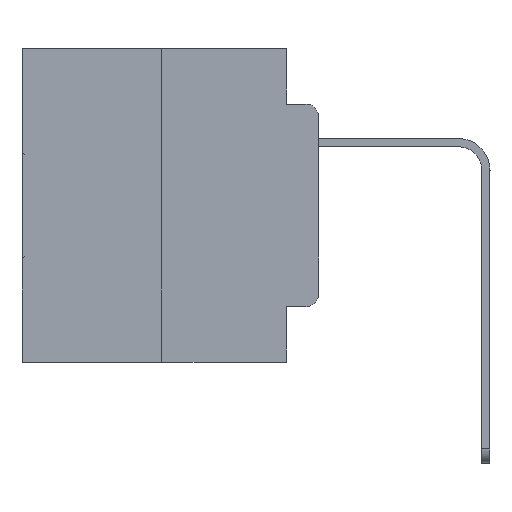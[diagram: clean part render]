
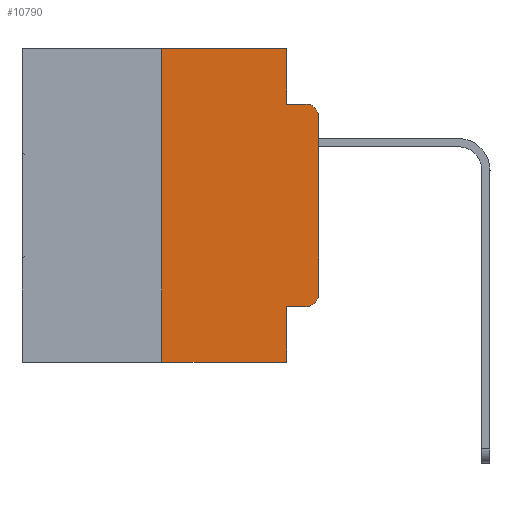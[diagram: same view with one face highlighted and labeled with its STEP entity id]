
A CAD part, left-side view. The second image highlights one B-rep face of the part: STEP entity #10790.
In plain terms, the highlighted planar face has unit normal (-1, 0, 0).
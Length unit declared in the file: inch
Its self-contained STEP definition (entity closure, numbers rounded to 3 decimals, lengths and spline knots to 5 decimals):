
#261 = EDGE_CURVE ( 'NONE', #13056, #20516, #25706, .T. ) ;
#331 = DIRECTION ( 'NONE',  ( 0., -1., 0. ) ) ;
#450 = LINE ( 'NONE', #11831, #4779 ) ;
#1232 = ORIENTED_EDGE ( 'NONE', *, *, #9289, .T. ) ;
#1322 = CARTESIAN_POINT ( 'NONE',  ( 0., 0.051, -0.0885 ) ) ;
#1327 = DIRECTION ( 'NONE',  ( 0., 0., 1. ) ) ;
#1960 = CARTESIAN_POINT ( 'NONE',  ( 0., 0.473, 0. ) ) ;
#2328 = CARTESIAN_POINT ( 'NONE',  ( 0., 0.473, 0. ) ) ;
#2825 = DIRECTION ( 'NONE',  ( 0., 0., 1. ) ) ;
#2968 = CIRCLE ( 'NONE', #25870, 0.02 ) ;
#3244 = DIRECTION ( 'NONE',  ( 0., -1., 0. ) ) ;
#3782 = ORIENTED_EDGE ( 'NONE', *, *, #261, .T. ) ;
#4067 = AXIS2_PLACEMENT_3D ( 'NONE', #21794, #7957, #21689 ) ;
#4076 = DIRECTION ( 'NONE',  ( 0., 0., -1. ) ) ;
#4779 = VECTOR ( 'NONE', #25373, 39.37008 ) ;
#4971 = CIRCLE ( 'NONE', #4067, 0.02 ) ;
#5511 = VERTEX_POINT ( 'NONE', #26132 ) ;
#5815 = AXIS2_PLACEMENT_3D ( 'NONE', #1960, #29541, #8828 ) ;
#6284 = VERTEX_POINT ( 'NONE', #7393 ) ;
#6319 = LINE ( 'NONE', #12357, #19334 ) ;
#7393 = CARTESIAN_POINT ( 'NONE',  ( 0., 0., -0.3915 ) ) ;
#7795 = LINE ( 'NONE', #10802, #28072 ) ;
#7957 = DIRECTION ( 'NONE',  ( -1., 0., 0. ) ) ;
#8068 = CARTESIAN_POINT ( 'NONE',  ( 0., 0.051, -0.5 ) ) ;
#8568 = CARTESIAN_POINT ( 'NONE',  ( 0., 0., -0.1085 ) ) ;
#8631 = CARTESIAN_POINT ( 'NONE',  ( 0., 0.02, -0.1085 ) ) ;
#8828 = DIRECTION ( 'NONE',  ( 0., 0., -1. ) ) ;
#9289 = EDGE_CURVE ( 'NONE', #18850, #25964, #2968, .T. ) ;
#9648 = ORIENTED_EDGE ( 'NONE', *, *, #10209, .T. ) ;
#9759 = ORIENTED_EDGE ( 'NONE', *, *, #24060, .F. ) ;
#10209 = EDGE_CURVE ( 'NONE', #6284, #18850, #12291, .T. ) ;
#10250 = CARTESIAN_POINT ( 'NONE',  ( 0., 0.02, -0.0885 ) ) ;
#10572 = VERTEX_POINT ( 'NONE', #28753 ) ;
#10612 = CARTESIAN_POINT ( 'NONE',  ( 0., 0.051, -0.4115 ) ) ;
#10790 = ADVANCED_FACE ( 'NONE', ( #12600 ), #29660, .F. ) ;
#10802 = CARTESIAN_POINT ( 'NONE',  ( 0., 0.25, 0. ) ) ;
#11635 = LINE ( 'NONE', #2328, #15584 ) ;
#11815 = EDGE_CURVE ( 'NONE', #20516, #6284, #4971, .T. ) ;
#11831 = CARTESIAN_POINT ( 'NONE',  ( 0., 0.051, 0. ) ) ;
#12291 = LINE ( 'NONE', #28083, #13750 ) ;
#12319 = VERTEX_POINT ( 'NONE', #19251 ) ;
#12357 = CARTESIAN_POINT ( 'NONE',  ( 0., 0.051, 0. ) ) ;
#12488 = ORIENTED_EDGE ( 'NONE', *, *, #26448, .F. ) ;
#12600 = FACE_OUTER_BOUND ( 'NONE', #18421, .T. ) ;
#13056 = VERTEX_POINT ( 'NONE', #10612 ) ;
#13747 = ORIENTED_EDGE ( 'NONE', *, *, #19935, .T. ) ;
#13750 = VECTOR ( 'NONE', #2825, 39.37008 ) ;
#14629 = CARTESIAN_POINT ( 'NONE',  ( 0., 0.473, -0.5 ) ) ;
#15311 = ORIENTED_EDGE ( 'NONE', *, *, #15636, .F. ) ;
#15584 = VECTOR ( 'NONE', #331, 39.37008 ) ;
#15636 = EDGE_CURVE ( 'NONE', #10572, #5511, #7795, .T. ) ;
#15738 = ORIENTED_EDGE ( 'NONE', *, *, #23902, .F. ) ;
#16781 = CARTESIAN_POINT ( 'NONE',  ( 0., 0.051, -0.4115 ) ) ;
#16841 = DIRECTION ( 'NONE',  ( 0., -1., 0. ) ) ;
#18421 = EDGE_LOOP ( 'NONE', ( #9648, #1232, #9759, #20560, #15738, #15311, #13747, #12488, #3782, #26384 ) ) ;
#18489 = EDGE_CURVE ( 'NONE', #24319, #12319, #450, .T. ) ;
#18517 = DIRECTION ( 'NONE',  ( 0., 0., -1. ) ) ;
#18850 = VERTEX_POINT ( 'NONE', #8568 ) ;
#19240 = CARTESIAN_POINT ( 'NONE',  ( 0., 0.02, -0.4115 ) ) ;
#19251 = CARTESIAN_POINT ( 'NONE',  ( 0., 0.051, -0.0885 ) ) ;
#19334 = VECTOR ( 'NONE', #18517, 39.37008 ) ;
#19561 = VECTOR ( 'NONE', #23874, 39.37008 ) ;
#19935 = EDGE_CURVE ( 'NONE', #10572, #28666, #22360, .T. ) ;
#20392 = CARTESIAN_POINT ( 'NONE',  ( 0., 0.051, 0. ) ) ;
#20516 = VERTEX_POINT ( 'NONE', #19240 ) ;
#20560 = ORIENTED_EDGE ( 'NONE', *, *, #18489, .F. ) ;
#21689 = DIRECTION ( 'NONE',  ( 0., 0., -1. ) ) ;
#21794 = CARTESIAN_POINT ( 'NONE',  ( 0., 0.02, -0.3915 ) ) ;
#22252 = DIRECTION ( 'NONE',  ( -1., 0., 0. ) ) ;
#22360 = LINE ( 'NONE', #14629, #28887 ) ;
#23874 = DIRECTION ( 'NONE',  ( 0., -1., 0. ) ) ;
#23902 = EDGE_CURVE ( 'NONE', #5511, #24319, #11635, .T. ) ;
#24060 = EDGE_CURVE ( 'NONE', #12319, #25964, #29355, .T. ) ;
#24319 = VERTEX_POINT ( 'NONE', #20392 ) ;
#25373 = DIRECTION ( 'NONE',  ( 0., 0., -1. ) ) ;
#25706 = LINE ( 'NONE', #16781, #19561 ) ;
#25870 = AXIS2_PLACEMENT_3D ( 'NONE', #8631, #22252, #4076 ) ;
#25964 = VERTEX_POINT ( 'NONE', #10250 ) ;
#26132 = CARTESIAN_POINT ( 'NONE',  ( 0., 0.25, 0. ) ) ;
#26384 = ORIENTED_EDGE ( 'NONE', *, *, #11815, .T. ) ;
#26448 = EDGE_CURVE ( 'NONE', #13056, #28666, #6319, .T. ) ;
#27163 = VECTOR ( 'NONE', #3244, 39.37008 ) ;
#28072 = VECTOR ( 'NONE', #1327, 39.37008 ) ;
#28083 = CARTESIAN_POINT ( 'NONE',  ( 0., 0., 0. ) ) ;
#28666 = VERTEX_POINT ( 'NONE', #8068 ) ;
#28753 = CARTESIAN_POINT ( 'NONE',  ( 0., 0.25, -0.5 ) ) ;
#28887 = VECTOR ( 'NONE', #16841, 39.37008 ) ;
#29355 = LINE ( 'NONE', #1322, #27163 ) ;
#29541 = DIRECTION ( 'NONE',  ( 1., 0., 0. ) ) ;
#29660 = PLANE ( 'NONE',  #5815 ) ;
